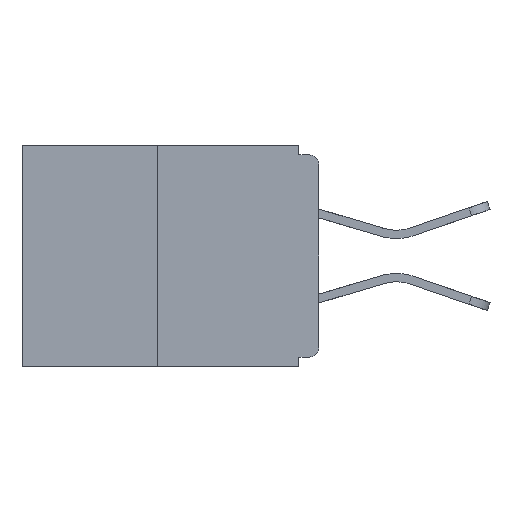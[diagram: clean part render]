
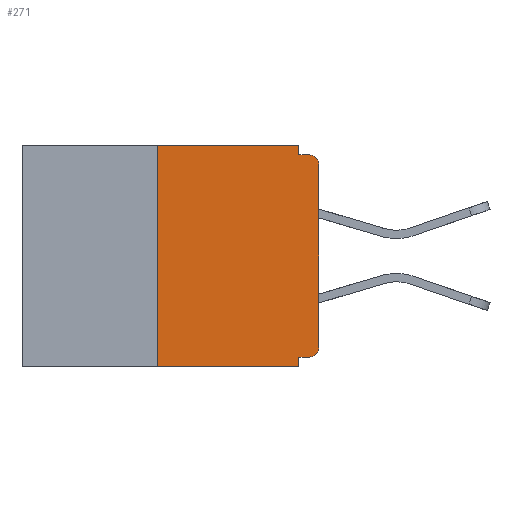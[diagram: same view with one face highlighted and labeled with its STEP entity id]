
A CAD part, left-side view. The second image highlights one B-rep face of the part: STEP entity #271.
In plain terms, the highlighted planar face has unit normal (-1, 0, 0).
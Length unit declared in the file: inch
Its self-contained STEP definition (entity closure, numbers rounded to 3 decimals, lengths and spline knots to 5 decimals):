
#188 = CARTESIAN_POINT ( 'NONE',  ( 0., 0.25, 0. ) ) ;
#271 = ADVANCED_FACE ( 'NONE', ( #14940 ), #25588, .F. ) ;
#544 = ORIENTED_EDGE ( 'NONE', *, *, #27834, .F. ) ;
#642 = AXIS2_PLACEMENT_3D ( 'NONE', #16925, #25279, #4049 ) ;
#1152 = CARTESIAN_POINT ( 'NONE',  ( 0., 0., -0.328 ) ) ;
#1322 = ORIENTED_EDGE ( 'NONE', *, *, #20629, .F. ) ;
#1609 = DIRECTION ( 'NONE',  ( 0., 0., -1. ) ) ;
#2706 = VERTEX_POINT ( 'NONE', #21140 ) ;
#2838 = CARTESIAN_POINT ( 'NONE',  ( 0., 0.031, -0.328 ) ) ;
#3146 = DIRECTION ( 'NONE',  ( -1., 0., 0. ) ) ;
#3370 = VECTOR ( 'NONE', #4642, 39.37008 ) ;
#3649 = CARTESIAN_POINT ( 'NONE',  ( 0., 0., -0.015 ) ) ;
#3839 = ORIENTED_EDGE ( 'NONE', *, *, #15997, .F. ) ;
#4049 = DIRECTION ( 'NONE',  ( 0., 0., -1. ) ) ;
#4531 = DIRECTION ( 'NONE',  ( 0., 0., 1. ) ) ;
#4642 = DIRECTION ( 'NONE',  ( 0., 0., -1. ) ) ;
#5324 = LINE ( 'NONE', #12270, #12708 ) ;
#5394 = LINE ( 'NONE', #19953, #3370 ) ;
#5410 = CARTESIAN_POINT ( 'NONE',  ( 0., 0.015, -0.03 ) ) ;
#5853 = CARTESIAN_POINT ( 'NONE',  ( 0., 0.031, -0.343 ) ) ;
#6425 = VERTEX_POINT ( 'NONE', #5853 ) ;
#6768 = ORIENTED_EDGE ( 'NONE', *, *, #9601, .T. ) ;
#6891 = CARTESIAN_POINT ( 'NONE',  ( 0., 0.015, -0.328 ) ) ;
#6900 = VECTOR ( 'NONE', #11086, 39.37008 ) ;
#7249 = CARTESIAN_POINT ( 'NONE',  ( 0., 0.46, 0. ) ) ;
#7305 = DIRECTION ( 'NONE',  ( 0., 0., -1. ) ) ;
#8218 = DIRECTION ( 'NONE',  ( 0., 0., 1. ) ) ;
#8256 = LINE ( 'NONE', #1152, #23381 ) ;
#8633 = EDGE_CURVE ( 'NONE', #17069, #2706, #12821, .T. ) ;
#8759 = VERTEX_POINT ( 'NONE', #18496 ) ;
#9394 = EDGE_CURVE ( 'NONE', #22108, #6425, #5394, .T. ) ;
#9601 = EDGE_CURVE ( 'NONE', #23647, #8759, #11435, .T. ) ;
#9613 = LINE ( 'NONE', #15840, #25423 ) ;
#10100 = ORIENTED_EDGE ( 'NONE', *, *, #16940, .T. ) ;
#11068 = LINE ( 'NONE', #3649, #21162 ) ;
#11086 = DIRECTION ( 'NONE',  ( 0., -1., 0. ) ) ;
#11380 = DIRECTION ( 'NONE',  ( 0., -1., 0. ) ) ;
#11435 = CIRCLE ( 'NONE', #642, 0.015 ) ;
#11526 = DIRECTION ( 'NONE',  ( 0., 0., -1. ) ) ;
#12069 = DIRECTION ( 'NONE',  ( 0., 1., 0. ) ) ;
#12270 = CARTESIAN_POINT ( 'NONE',  ( 0., 0., 0. ) ) ;
#12708 = VECTOR ( 'NONE', #8218, 39.37008 ) ;
#12821 = CIRCLE ( 'NONE', #17420, 0.015 ) ;
#13307 = ORIENTED_EDGE ( 'NONE', *, *, #8633, .T. ) ;
#13502 = CARTESIAN_POINT ( 'NONE',  ( 0., 0.46, -0.343 ) ) ;
#14214 = ORIENTED_EDGE ( 'NONE', *, *, #9394, .F. ) ;
#14712 = CARTESIAN_POINT ( 'NONE',  ( 0., 0.031, -0.015 ) ) ;
#14940 = FACE_OUTER_BOUND ( 'NONE', #20371, .T. ) ;
#15840 = CARTESIAN_POINT ( 'NONE',  ( 0., 0.031, 0. ) ) ;
#15997 = EDGE_CURVE ( 'NONE', #23647, #22108, #8256, .T. ) ;
#16607 = VERTEX_POINT ( 'NONE', #14712 ) ;
#16687 = AXIS2_PLACEMENT_3D ( 'NONE', #23237, #21090, #1609 ) ;
#16771 = VERTEX_POINT ( 'NONE', #23028 ) ;
#16925 = CARTESIAN_POINT ( 'NONE',  ( 0., 0.015, -0.313 ) ) ;
#16940 = EDGE_CURVE ( 'NONE', #27320, #6425, #24020, .T. ) ;
#17069 = VERTEX_POINT ( 'NONE', #21557 ) ;
#17420 = AXIS2_PLACEMENT_3D ( 'NONE', #5410, #3146, #11526 ) ;
#17864 = EDGE_CURVE ( 'NONE', #8759, #17069, #5324, .T. ) ;
#18496 = CARTESIAN_POINT ( 'NONE',  ( 0., 0., -0.313 ) ) ;
#18629 = VERTEX_POINT ( 'NONE', #26979 ) ;
#19953 = CARTESIAN_POINT ( 'NONE',  ( 0., 0.031, -0.343 ) ) ;
#20247 = ORIENTED_EDGE ( 'NONE', *, *, #20840, .F. ) ;
#20306 = LINE ( 'NONE', #188, #25342 ) ;
#20371 = EDGE_LOOP ( 'NONE', ( #20247, #1322, #10100, #14214, #3839, #6768, #24099, #13307, #23422, #544 ) ) ;
#20629 = EDGE_CURVE ( 'NONE', #27320, #18629, #20306, .T. ) ;
#20840 = EDGE_CURVE ( 'NONE', #18629, #16771, #22962, .T. ) ;
#20957 = DIRECTION ( 'NONE',  ( 0., -1., 0. ) ) ;
#21090 = DIRECTION ( 'NONE',  ( 1., 0., 0. ) ) ;
#21140 = CARTESIAN_POINT ( 'NONE',  ( 0., 0.015, -0.015 ) ) ;
#21162 = VECTOR ( 'NONE', #20957, 39.37008 ) ;
#21557 = CARTESIAN_POINT ( 'NONE',  ( 0., 0., -0.03 ) ) ;
#22108 = VERTEX_POINT ( 'NONE', #2838 ) ;
#22962 = LINE ( 'NONE', #7249, #27322 ) ;
#23028 = CARTESIAN_POINT ( 'NONE',  ( 0., 0.031, 0. ) ) ;
#23237 = CARTESIAN_POINT ( 'NONE',  ( 0., 0.46, 0. ) ) ;
#23381 = VECTOR ( 'NONE', #12069, 39.37008 ) ;
#23422 = ORIENTED_EDGE ( 'NONE', *, *, #26705, .F. ) ;
#23647 = VERTEX_POINT ( 'NONE', #6891 ) ;
#23967 = CARTESIAN_POINT ( 'NONE',  ( 0., 0.25, -0.343 ) ) ;
#24020 = LINE ( 'NONE', #13502, #6900 ) ;
#24099 = ORIENTED_EDGE ( 'NONE', *, *, #17864, .T. ) ;
#25279 = DIRECTION ( 'NONE',  ( -1., 0., 0. ) ) ;
#25342 = VECTOR ( 'NONE', #4531, 39.37008 ) ;
#25423 = VECTOR ( 'NONE', #7305, 39.37008 ) ;
#25588 = PLANE ( 'NONE',  #16687 ) ;
#26705 = EDGE_CURVE ( 'NONE', #16607, #2706, #11068, .T. ) ;
#26979 = CARTESIAN_POINT ( 'NONE',  ( 0., 0.25, 0. ) ) ;
#27320 = VERTEX_POINT ( 'NONE', #23967 ) ;
#27322 = VECTOR ( 'NONE', #11380, 39.37008 ) ;
#27834 = EDGE_CURVE ( 'NONE', #16771, #16607, #9613, .T. ) ;
